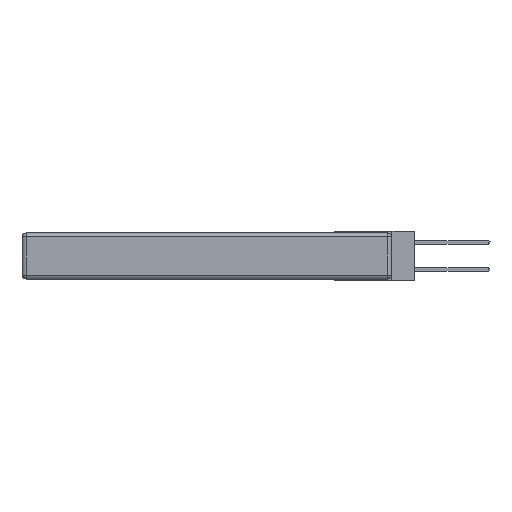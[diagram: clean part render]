
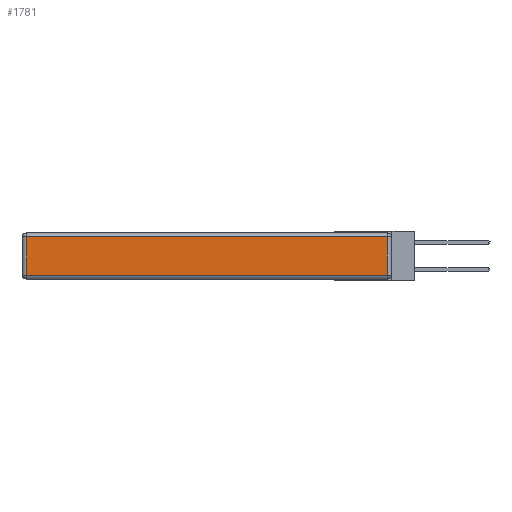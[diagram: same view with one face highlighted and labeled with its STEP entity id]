
A CAD part, left-side view. The second image highlights one B-rep face of the part: STEP entity #1781.
In plain terms, the highlighted planar face has unit normal (-1, 0, 0).
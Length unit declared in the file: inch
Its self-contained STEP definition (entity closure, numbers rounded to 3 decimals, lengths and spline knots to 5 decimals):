
#275 = CARTESIAN_POINT ( 'NONE',  ( 0., 0., -0.313 ) ) ;
#615 = VECTOR ( 'NONE', #7492, 39.37008 ) ;
#1436 = CARTESIAN_POINT ( 'NONE',  ( 0., 2.72, -0.03 ) ) ;
#1570 = CARTESIAN_POINT ( 'NONE',  ( 0., 0.03, -0.03 ) ) ;
#1696 = CARTESIAN_POINT ( 'NONE',  ( 0., 2.72, -0.343 ) ) ;
#1781 = ADVANCED_FACE ( 'NONE', ( #21235 ), #17104, .T. ) ;
#1966 = EDGE_CURVE ( 'NONE', #6200, #13194, #21813, .T. ) ;
#4067 = LINE ( 'NONE', #275, #615 ) ;
#4250 = DIRECTION ( 'NONE',  ( 0., 1., 0. ) ) ;
#5883 = EDGE_LOOP ( 'NONE', ( #16434, #20249, #22517, #10295 ) ) ;
#6051 = DIRECTION ( 'NONE',  ( -1., 0., 0. ) ) ;
#6200 = VERTEX_POINT ( 'NONE', #1570 ) ;
#7492 = DIRECTION ( 'NONE',  ( 0., -1., 0. ) ) ;
#7823 = CARTESIAN_POINT ( 'NONE',  ( 0., 0., -0.343 ) ) ;
#9953 = VECTOR ( 'NONE', #20216, 39.37008 ) ;
#10295 = ORIENTED_EDGE ( 'NONE', *, *, #16531, .T. ) ;
#10736 = AXIS2_PLACEMENT_3D ( 'NONE', #7823, #6051, #14100 ) ;
#11405 = VECTOR ( 'NONE', #14612, 39.37008 ) ;
#12809 = VERTEX_POINT ( 'NONE', #19579 ) ;
#13194 = VERTEX_POINT ( 'NONE', #1436 ) ;
#13329 = EDGE_CURVE ( 'NONE', #12809, #22701, #4067, .T. ) ;
#14033 = LINE ( 'NONE', #14599, #9953 ) ;
#14100 = DIRECTION ( 'NONE',  ( 0., 0., 1. ) ) ;
#14599 = CARTESIAN_POINT ( 'NONE',  ( 0., 0.03, -0.343 ) ) ;
#14612 = DIRECTION ( 'NONE',  ( 0., 0., -1. ) ) ;
#15379 = EDGE_CURVE ( 'NONE', #22701, #6200, #14033, .T. ) ;
#16434 = ORIENTED_EDGE ( 'NONE', *, *, #13329, .T. ) ;
#16531 = EDGE_CURVE ( 'NONE', #13194, #12809, #17799, .T. ) ;
#17104 = PLANE ( 'NONE',  #10736 ) ;
#17799 = LINE ( 'NONE', #1696, #11405 ) ;
#19104 = CARTESIAN_POINT ( 'NONE',  ( 0., 2.75, -0.03 ) ) ;
#19188 = VECTOR ( 'NONE', #4250, 39.37008 ) ;
#19579 = CARTESIAN_POINT ( 'NONE',  ( 0., 2.72, -0.313 ) ) ;
#20216 = DIRECTION ( 'NONE',  ( 0., 0., 1. ) ) ;
#20249 = ORIENTED_EDGE ( 'NONE', *, *, #15379, .T. ) ;
#21235 = FACE_OUTER_BOUND ( 'NONE', #5883, .T. ) ;
#21706 = CARTESIAN_POINT ( 'NONE',  ( 0., 0.03, -0.313 ) ) ;
#21813 = LINE ( 'NONE', #19104, #19188 ) ;
#22517 = ORIENTED_EDGE ( 'NONE', *, *, #1966, .T. ) ;
#22701 = VERTEX_POINT ( 'NONE', #21706 ) ;
